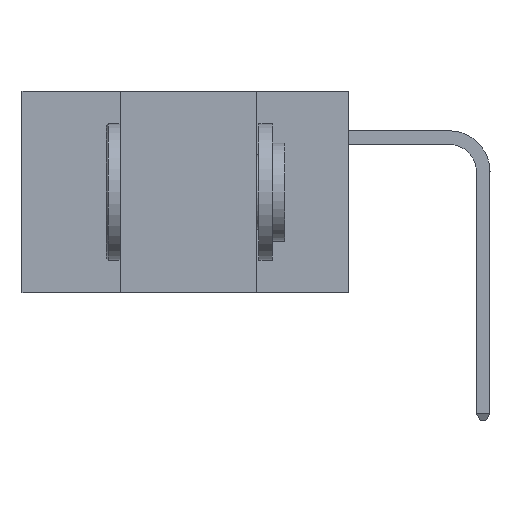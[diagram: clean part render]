
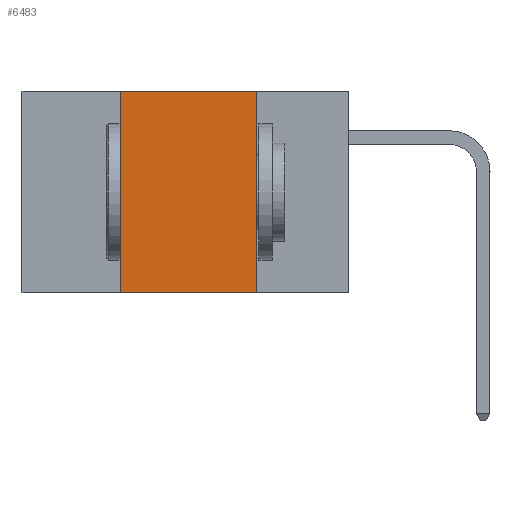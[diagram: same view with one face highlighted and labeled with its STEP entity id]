
A CAD part, left-side view. The second image highlights one B-rep face of the part: STEP entity #6483.
In plain terms, the highlighted planar face has unit normal (-1, 0, 0).
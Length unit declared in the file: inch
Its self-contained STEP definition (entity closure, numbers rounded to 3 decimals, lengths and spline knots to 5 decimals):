
#1190 = DIRECTION ( 'NONE',  ( 0., 0., -1. ) ) ;
#1401 = LINE ( 'NONE', #7220, #4194 ) ;
#1435 = DIRECTION ( 'NONE',  ( 0., 0., 1. ) ) ;
#1623 = EDGE_LOOP ( 'NONE', ( #14269, #10809, #11335, #10640 ) ) ;
#1806 = LINE ( 'NONE', #9374, #14225 ) ;
#2017 = CARTESIAN_POINT ( 'NONE',  ( 0., 0.17, 0. ) ) ;
#2274 = CARTESIAN_POINT ( 'NONE',  ( 0., 0.42, 0. ) ) ;
#2387 = AXIS2_PLACEMENT_3D ( 'NONE', #15145, #8355, #1190 ) ;
#2905 = VECTOR ( 'NONE', #1435, 39.37008 ) ;
#3546 = EDGE_CURVE ( 'NONE', #3801, #6593, #1401, .T. ) ;
#3801 = VERTEX_POINT ( 'NONE', #2017 ) ;
#3979 = DIRECTION ( 'NONE',  ( 0., -1., 0. ) ) ;
#4194 = VECTOR ( 'NONE', #4688, 39.37008 ) ;
#4688 = DIRECTION ( 'NONE',  ( 0., 0., -1. ) ) ;
#6379 = CARTESIAN_POINT ( 'NONE',  ( 0., 0.6, 0. ) ) ;
#6483 = ADVANCED_FACE ( 'NONE', ( #14757 ), #12895, .F. ) ;
#6593 = VERTEX_POINT ( 'NONE', #7387 ) ;
#6692 = EDGE_CURVE ( 'NONE', #9717, #3801, #9639, .T. ) ;
#7157 = EDGE_CURVE ( 'NONE', #11276, #9717, #14913, .T. ) ;
#7220 = CARTESIAN_POINT ( 'NONE',  ( 0., 0.17, 0. ) ) ;
#7387 = CARTESIAN_POINT ( 'NONE',  ( 0., 0.17, -0.37 ) ) ;
#8355 = DIRECTION ( 'NONE',  ( 1., 0., 0. ) ) ;
#9374 = CARTESIAN_POINT ( 'NONE',  ( 0., 0.6, -0.37 ) ) ;
#9639 = LINE ( 'NONE', #6379, #14927 ) ;
#9717 = VERTEX_POINT ( 'NONE', #2274 ) ;
#10529 = DIRECTION ( 'NONE',  ( 0., -1., 0. ) ) ;
#10640 = ORIENTED_EDGE ( 'NONE', *, *, #11528, .T. ) ;
#10809 = ORIENTED_EDGE ( 'NONE', *, *, #6692, .F. ) ;
#10923 = CARTESIAN_POINT ( 'NONE',  ( 0., 0.42, 0. ) ) ;
#11276 = VERTEX_POINT ( 'NONE', #14697 ) ;
#11335 = ORIENTED_EDGE ( 'NONE', *, *, #7157, .F. ) ;
#11528 = EDGE_CURVE ( 'NONE', #11276, #6593, #1806, .T. ) ;
#12895 = PLANE ( 'NONE',  #2387 ) ;
#14225 = VECTOR ( 'NONE', #10529, 39.37008 ) ;
#14269 = ORIENTED_EDGE ( 'NONE', *, *, #3546, .F. ) ;
#14697 = CARTESIAN_POINT ( 'NONE',  ( 0., 0.42, -0.37 ) ) ;
#14757 = FACE_OUTER_BOUND ( 'NONE', #1623, .T. ) ;
#14913 = LINE ( 'NONE', #10923, #2905 ) ;
#14927 = VECTOR ( 'NONE', #3979, 39.37008 ) ;
#15145 = CARTESIAN_POINT ( 'NONE',  ( 0., 0.6, 0. ) ) ;
